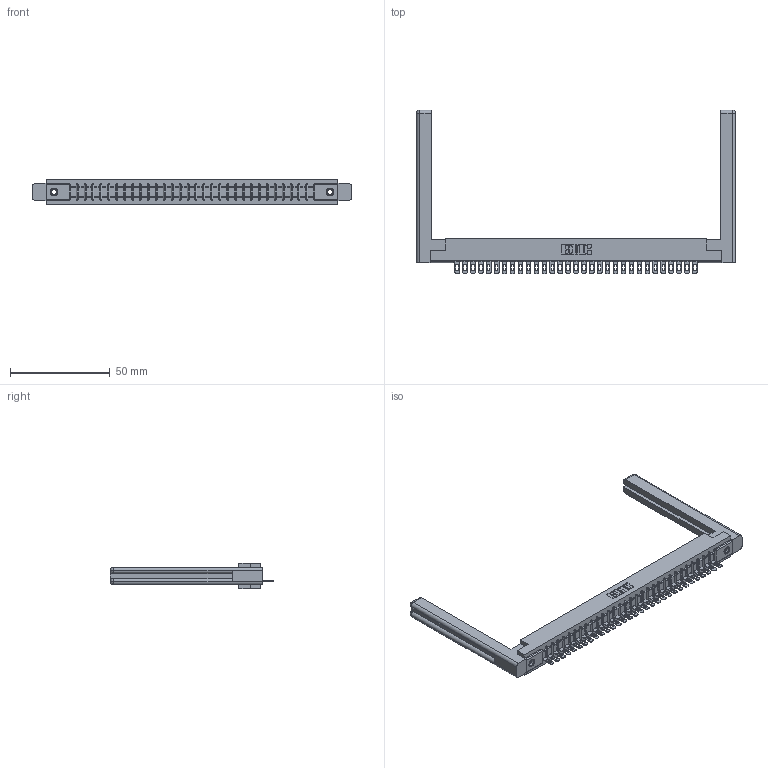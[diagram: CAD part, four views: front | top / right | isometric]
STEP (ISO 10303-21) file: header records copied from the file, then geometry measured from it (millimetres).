
FILE_DESCRIPTION (( 'STEP AP203' ), '1' );
FILE_NAME ('307-031-401-158.STEP', '2020-09-28T13:55:35', ( '' ), ( '' ), 'SwSTEP 2.0', 'SolidWorks 2020', '' );
FILE_SCHEMA (( 'CONFIG_CONTROL_DESIGN' ));
Length unit declared in the file: inch
Products named in the file (5): 307 Part_.156 Dia Mounting Holes; 307-290-002_501; 307-220-058; 345-250-001_345-250-001-102; 307-031-401-158
Assembly tree (36 placements, depth 2):
  307-031-401-158
    307 Part_.156 Dia Mounting Holes
    307-290-002_501  x31
    307-220-058  x2
    345-250-001_345-250-001-102  x2
Bounding box: 159.46 x 81.74 x 12.7 mm (x, y, z)
Volume: 24129.6 mm3; surface area: 26187.2 mm2
Topology: 36 solids, 36 shells, 2648 faces, 8055 edges, 5270 vertices
Faces by surface type: plane 1518, cylinder 1042, sphere 64, torus 12, cone 12
Entity records: 31359 total; most frequent: CARTESIAN_POINT 5295, ORIENTED_EDGE 5224, DIRECTION 5114, EDGE_CURVE 2612, VECTOR 1988, LINE 1988, VERTEX_POINT 1690, AXIS2_PLACEMENT_3D 1563
